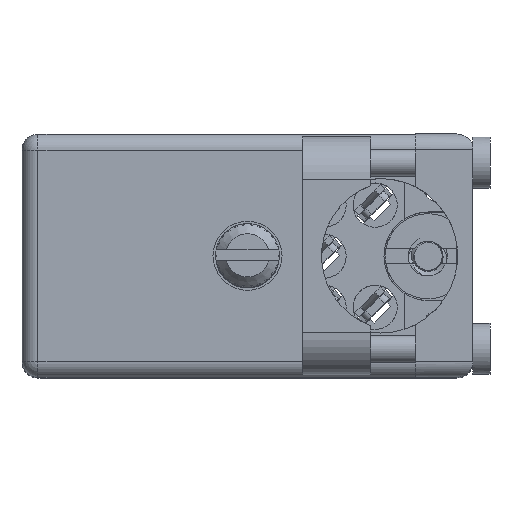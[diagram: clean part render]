
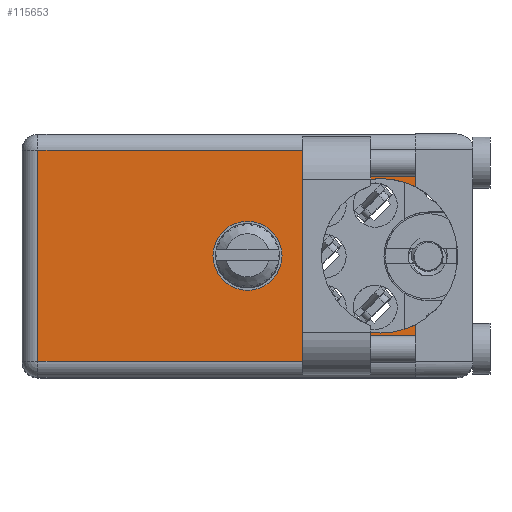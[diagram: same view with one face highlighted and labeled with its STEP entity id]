
A CAD part, top view. The second image highlights one B-rep face of the part: STEP entity #115653.
In plain terms, the highlighted face is planar.
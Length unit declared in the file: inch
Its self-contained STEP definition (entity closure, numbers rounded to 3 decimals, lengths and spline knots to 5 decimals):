
#725 = CARTESIAN_POINT ( 'NONE',  ( 0., 0.906, -0.715 ) ) ;
#4599 = CARTESIAN_POINT ( 'NONE',  ( 1.155, 0.906, 0. ) ) ;
#9046 = VERTEX_POINT ( 'NONE', #63913 ) ;
#11187 = CARTESIAN_POINT ( 'NONE',  ( 1.053, 0.906, -0.1305 ) ) ;
#11717 = AXIS2_PLACEMENT_3D ( 'NONE', #725, #31012, #165982 ) ;
#13487 = CARTESIAN_POINT ( 'NONE',  ( 1.155, 0.906, -0.15471 ) ) ;
#16512 = EDGE_CURVE ( 'NONE', #9046, #173224, #168645, .T. ) ;
#19376 = VERTEX_POINT ( 'NONE', #162571 ) ;
#23835 = ORIENTED_EDGE ( 'NONE', *, *, #33625, .F. ) ;
#26602 = DIRECTION ( 'NONE',  ( 0., 0., 1. ) ) ;
#31012 = DIRECTION ( 'NONE',  ( 0., 1., 0. ) ) ;
#31491 = EDGE_CURVE ( 'NONE', #100466, #184362, #115791, .T. ) ;
#31911 = CARTESIAN_POINT ( 'NONE',  ( 0.047, 0.906, -0.715 ) ) ;
#33310 = CIRCLE ( 'NONE', #161833, 0.227 ) ;
#33625 = EDGE_CURVE ( 'NONE', #173224, #125615, #33310, .T. ) ;
#37860 = ORIENTED_EDGE ( 'NONE', *, *, #140644, .F. ) ;
#42252 = DIRECTION ( 'NONE',  ( 0., 1., 0. ) ) ;
#45738 = DIRECTION ( 'NONE',  ( 0., 0., 1. ) ) ;
#45765 = ORIENTED_EDGE ( 'NONE', *, *, #98394, .F. ) ;
#49174 = VECTOR ( 'NONE', #45738, 39.37008 ) ;
#50698 = CARTESIAN_POINT ( 'NONE',  ( 0., 0.906, -0.668 ) ) ;
#52909 = CIRCLE ( 'NONE', #80552, 0.1015 ) ;
#56523 = LINE ( 'NONE', #50698, #122480 ) ;
#57085 = ORIENTED_EDGE ( 'NONE', *, *, #162467, .F. ) ;
#57952 = DIRECTION ( 'NONE',  ( 0., 0., 1. ) ) ;
#59740 = DIRECTION ( 'NONE',  ( 0., 1., 0. ) ) ;
#59944 = VERTEX_POINT ( 'NONE', #145844 ) ;
#61727 = LINE ( 'NONE', #87682, #66426 ) ;
#61814 = EDGE_CURVE ( 'NONE', #171835, #9046, #172114, .T. ) ;
#63913 = CARTESIAN_POINT ( 'NONE',  ( 1.053, 0.906, -0.5845 ) ) ;
#66426 = VECTOR ( 'NONE', #114845, 39.37008 ) ;
#68955 = LINE ( 'NONE', #144207, #144362 ) ;
#72000 = CARTESIAN_POINT ( 'NONE',  ( 0.047, 0.906, -0.668 ) ) ;
#72504 = EDGE_CURVE ( 'NONE', #80149, #19376, #61727, .T. ) ;
#72841 = CARTESIAN_POINT ( 'NONE',  ( 1.053, 0.906, -0.3575 ) ) ;
#74385 = ORIENTED_EDGE ( 'NONE', *, *, #72504, .T. ) ;
#74474 = ORIENTED_EDGE ( 'NONE', *, *, #77870, .T. ) ;
#75170 = EDGE_LOOP ( 'NONE', ( #57085, #144494, #74474, #74385, #45765, #23835, #84957, #82472 ) ) ;
#76110 = EDGE_CURVE ( 'NONE', #59944, #113912, #56523, .T. ) ;
#77870 = EDGE_CURVE ( 'NONE', #113912, #80149, #112812, .T. ) ;
#78702 = FACE_BOUND ( 'NONE', #102033, .T. ) ;
#80149 = VERTEX_POINT ( 'NONE', #113377 ) ;
#80552 = AXIS2_PLACEMENT_3D ( 'NONE', #163532, #102858, #26602 ) ;
#82472 = ORIENTED_EDGE ( 'NONE', *, *, #61814, .F. ) ;
#82576 = VECTOR ( 'NONE', #111825, 39.37008 ) ;
#84957 = ORIENTED_EDGE ( 'NONE', *, *, #16512, .F. ) ;
#87682 = CARTESIAN_POINT ( 'NONE',  ( 1.155, 0.906, -0.047 ) ) ;
#94244 = LINE ( 'NONE', #4599, #82576 ) ;
#98394 = EDGE_CURVE ( 'NONE', #125615, #19376, #94244, .T. ) ;
#100466 = VERTEX_POINT ( 'NONE', #119446 ) ;
#102033 = EDGE_LOOP ( 'NONE', ( #37860, #145855 ) ) ;
#102858 = DIRECTION ( 'NONE',  ( 0., 1., 0. ) ) ;
#103218 = DIRECTION ( 'NONE',  ( 0., 0., 1. ) ) ;
#103391 = AXIS2_PLACEMENT_3D ( 'NONE', #105883, #121105, #136233 ) ;
#104018 = CARTESIAN_POINT ( 'NONE',  ( 0.6625, 0.906, -0.3575 ) ) ;
#105883 = CARTESIAN_POINT ( 'NONE',  ( 1.053, 0.906, -0.3575 ) ) ;
#107642 = DIRECTION ( 'NONE',  ( 0., 0., 1. ) ) ;
#111825 = DIRECTION ( 'NONE',  ( 0., 0., 1. ) ) ;
#112812 = LINE ( 'NONE', #31911, #49174 ) ;
#113377 = CARTESIAN_POINT ( 'NONE',  ( 0.047, 0.906, -0.047 ) ) ;
#113912 = VERTEX_POINT ( 'NONE', #72000 ) ;
#114081 = FACE_OUTER_BOUND ( 'NONE', #75170, .T. ) ;
#114845 = DIRECTION ( 'NONE',  ( 1., 0., 0. ) ) ;
#115653 = ADVANCED_FACE ( 'NONE', ( #114081, #78702 ), #167264, .T. ) ;
#115791 = CIRCLE ( 'NONE', #128580, 0.1015 ) ;
#118329 = DIRECTION ( 'NONE',  ( 0., 1., 0. ) ) ;
#119446 = CARTESIAN_POINT ( 'NONE',  ( 0.6625, 0.906, -0.459 ) ) ;
#121105 = DIRECTION ( 'NONE',  ( 0., 1., 0. ) ) ;
#122480 = VECTOR ( 'NONE', #156702, 39.37008 ) ;
#125615 = VERTEX_POINT ( 'NONE', #13487 ) ;
#128580 = AXIS2_PLACEMENT_3D ( 'NONE', #104018, #42252, #57952 ) ;
#132800 = CARTESIAN_POINT ( 'NONE',  ( 1.155, 0.906, -0.56029 ) ) ;
#135200 = CARTESIAN_POINT ( 'NONE',  ( 0.6625, 0.906, -0.256 ) ) ;
#136233 = DIRECTION ( 'NONE',  ( 0., 0., 1. ) ) ;
#140644 = EDGE_CURVE ( 'NONE', #184362, #100466, #52909, .T. ) ;
#144207 = CARTESIAN_POINT ( 'NONE',  ( 1.155, 0.906, 0. ) ) ;
#144362 = VECTOR ( 'NONE', #174542, 39.37008 ) ;
#144494 = ORIENTED_EDGE ( 'NONE', *, *, #76110, .T. ) ;
#145844 = CARTESIAN_POINT ( 'NONE',  ( 1.155, 0.906, -0.668 ) ) ;
#145855 = ORIENTED_EDGE ( 'NONE', *, *, #31491, .F. ) ;
#150614 = CARTESIAN_POINT ( 'NONE',  ( 1.053, 0.906, -0.3575 ) ) ;
#156702 = DIRECTION ( 'NONE',  ( -1., 0., 0. ) ) ;
#161833 = AXIS2_PLACEMENT_3D ( 'NONE', #150614, #59740, #103218 ) ;
#162467 = EDGE_CURVE ( 'NONE', #59944, #171835, #68955, .T. ) ;
#162571 = CARTESIAN_POINT ( 'NONE',  ( 1.155, 0.906, -0.047 ) ) ;
#163532 = CARTESIAN_POINT ( 'NONE',  ( 0.6625, 0.906, -0.3575 ) ) ;
#165982 = DIRECTION ( 'NONE',  ( 0., 0., 1. ) ) ;
#167264 = PLANE ( 'NONE',  #11717 ) ;
#168645 = CIRCLE ( 'NONE', #176431, 0.227 ) ;
#171835 = VERTEX_POINT ( 'NONE', #132800 ) ;
#172114 = CIRCLE ( 'NONE', #103391, 0.227 ) ;
#173224 = VERTEX_POINT ( 'NONE', #11187 ) ;
#174542 = DIRECTION ( 'NONE',  ( 0., 0., 1. ) ) ;
#176431 = AXIS2_PLACEMENT_3D ( 'NONE', #72841, #118329, #107642 ) ;
#184362 = VERTEX_POINT ( 'NONE', #135200 ) ;
